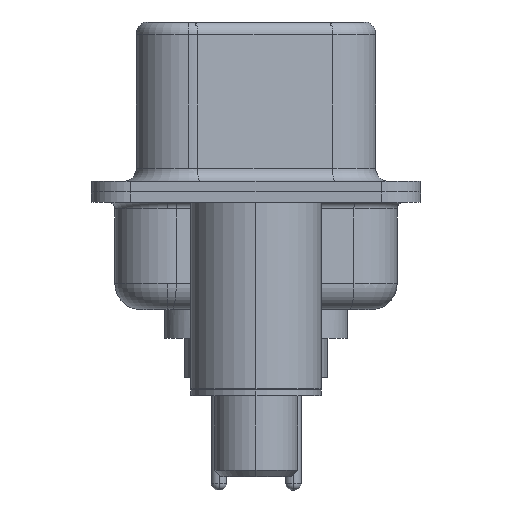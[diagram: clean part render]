
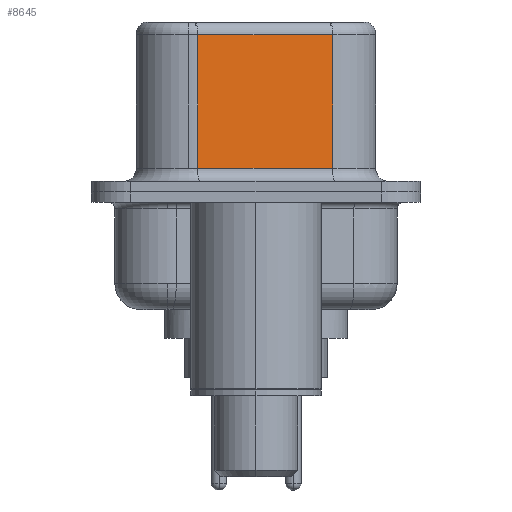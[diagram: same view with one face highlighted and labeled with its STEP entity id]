
A CAD part, left-side view. The second image highlights one B-rep face of the part: STEP entity #8645.
In plain terms, the highlighted planar face has unit normal (-0.985, -0.174, 0).
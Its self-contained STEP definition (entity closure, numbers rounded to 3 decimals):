
#804 = DIRECTION ( 'NONE',  ( -0.174, 0.985, 0. ) ) ;
#918 = LINE ( 'NONE', #19395, #22340 ) ;
#1286 = VECTOR ( 'NONE', #18552, 1000. ) ;
#1944 = CARTESIAN_POINT ( 'NONE',  ( 4.58, -2.927, 6.02 ) ) ;
#2596 = VERTEX_POINT ( 'NONE', #18213 ) ;
#5457 = EDGE_CURVE ( 'NONE', #7271, #2596, #918, .T. ) ;
#5790 = CARTESIAN_POINT ( 'NONE',  ( 3.67, 2.233, 6.02 ) ) ;
#6002 = CARTESIAN_POINT ( 'NONE',  ( 4.58, -2.927, 6.02 ) ) ;
#6747 = CARTESIAN_POINT ( 'NONE',  ( 4.58, -2.927, 6.52 ) ) ;
#6802 = LINE ( 'NONE', #6002, #1286 ) ;
#7271 = VERTEX_POINT ( 'NONE', #5790 ) ;
#8645 = ADVANCED_FACE ( 'NONE', ( #22916 ), #25656, .F. ) ;
#8833 = DIRECTION ( 'NONE',  ( 0., 0., -1. ) ) ;
#9040 = DIRECTION ( 'NONE',  ( 0.174, -0.985, 0. ) ) ;
#10331 = VECTOR ( 'NONE', #9040, 1000. ) ;
#11154 = CARTESIAN_POINT ( 'NONE',  ( 4.58, -2.927, 6.52 ) ) ;
#12242 = VECTOR ( 'NONE', #8833, 1000. ) ;
#12897 = ORIENTED_EDGE ( 'NONE', *, *, #26146, .T. ) ;
#13264 = DIRECTION ( 'NONE',  ( 0.985, 0.174, 0. ) ) ;
#14369 = AXIS2_PLACEMENT_3D ( 'NONE', #11154, #13264, #804 ) ;
#15749 = EDGE_CURVE ( 'NONE', #2596, #19916, #16549, .T. ) ;
#15915 = EDGE_LOOP ( 'NONE', ( #16117, #12897, #20024, #18797 ) ) ;
#16117 = ORIENTED_EDGE ( 'NONE', *, *, #16241, .F. ) ;
#16241 = EDGE_CURVE ( 'NONE', #25786, #19916, #19118, .T. ) ;
#16549 = LINE ( 'NONE', #21466, #10331 ) ;
#18213 = CARTESIAN_POINT ( 'NONE',  ( 3.67, 2.233, 0.9 ) ) ;
#18552 = DIRECTION ( 'NONE',  ( -0.174, 0.985, 0. ) ) ;
#18797 = ORIENTED_EDGE ( 'NONE', *, *, #15749, .T. ) ;
#19117 = DIRECTION ( 'NONE',  ( 0., 0., -1. ) ) ;
#19118 = LINE ( 'NONE', #6747, #12242 ) ;
#19395 = CARTESIAN_POINT ( 'NONE',  ( 3.67, 2.233, 6.52 ) ) ;
#19916 = VERTEX_POINT ( 'NONE', #26871 ) ;
#20024 = ORIENTED_EDGE ( 'NONE', *, *, #5457, .T. ) ;
#21466 = CARTESIAN_POINT ( 'NONE',  ( 4.58, -2.927, 0.9 ) ) ;
#22340 = VECTOR ( 'NONE', #19117, 1000. ) ;
#22916 = FACE_OUTER_BOUND ( 'NONE', #15915, .T. ) ;
#25656 = PLANE ( 'NONE',  #14369 ) ;
#25786 = VERTEX_POINT ( 'NONE', #1944 ) ;
#26146 = EDGE_CURVE ( 'NONE', #25786, #7271, #6802, .T. ) ;
#26871 = CARTESIAN_POINT ( 'NONE',  ( 4.58, -2.927, 0.9 ) ) ;
